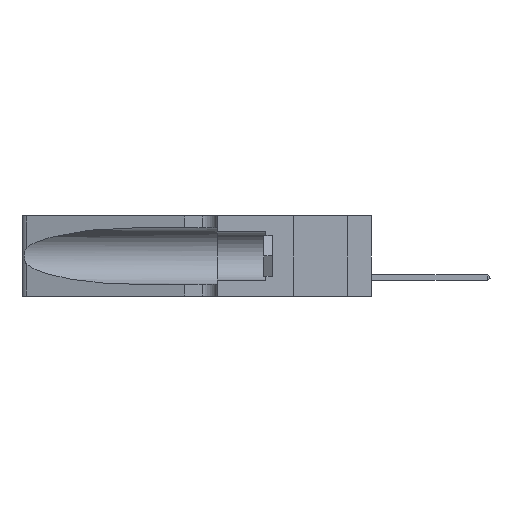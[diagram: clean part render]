
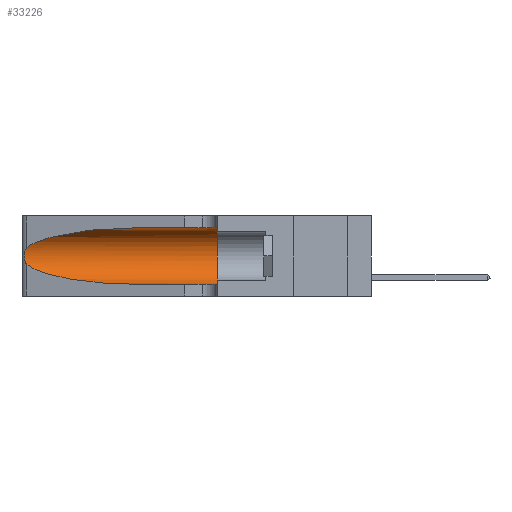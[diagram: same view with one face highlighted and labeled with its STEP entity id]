
A CAD part, left-side view. The second image highlights one B-rep face of the part: STEP entity #33226.
In plain terms, the highlighted cylindrical face has radius 3.308 mm (diameter 6.617 mm), a partial arc.
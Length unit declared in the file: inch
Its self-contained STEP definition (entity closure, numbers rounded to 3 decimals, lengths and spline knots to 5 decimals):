
#1278 = VERTEX_POINT ( 'NONE', #46199 ) ;
#1448 = CARTESIAN_POINT ( 'NONE',  ( 0.25555, 1.22993, 0.14849 ) ) ;
#1820 = CARTESIAN_POINT ( 'NONE',  ( 0.25555, 1.22994, 0.2215 ) ) ;
#1903 = CARTESIAN_POINT ( 'NONE',  ( 0.2373, 1.15595, 0.08982 ) ) ;
#3109 = CARTESIAN_POINT ( 'NONE',  ( 0.25487, 1.22718, 0.14631 ) ) ;
#5463 = CARTESIAN_POINT ( 'NONE',  ( 0.25789, 1.23486, 0.15765 ) ) ;
#5542 = CARTESIAN_POINT ( 'NONE',  ( 0.25487, 1.22718, 0.22369 ) ) ;
#6098 = VERTEX_POINT ( 'NONE', #3109 ) ;
#6198 = CARTESIAN_POINT ( 'NONE',  ( 0.26075, 1.23896, 0.19203 ) ) ;
#7115 = CARTESIAN_POINT ( 'NONE',  ( 0.25487, 1.22718, 0.22369 ) ) ;
#7576 = VERTEX_POINT ( 'NONE', #30046 ) ;
#7947 = CARTESIAN_POINT ( 'NONE',  ( 0.1305, 1.61858, 0.31525 ) ) ;
#8960 = ORIENTED_EDGE ( 'NONE', *, *, #21991, .T. ) ;
#10146 = CARTESIAN_POINT ( 'NONE',  ( 0.26075, 1.23896, 0.178 ) ) ;
#12109 = DIRECTION ( 'NONE',  ( 0., 1., 0. ) ) ;
#12801 = EDGE_CURVE ( 'NONE', #7576, #27896, #23315, .T. ) ;
#13102 = ORIENTED_EDGE ( 'NONE', *, *, #45933, .F. ) ;
#13615 = DIRECTION ( 'NONE',  ( 0., 0., -1. ) ) ;
#14048 = CARTESIAN_POINT ( 'NONE',  ( 0.25487, 1.22718, 0.22369 ) ) ;
#16147 = CARTESIAN_POINT ( 'NONE',  ( 0.1305, 0.72297, 0.31525 ) ) ;
#16413 = EDGE_CURVE ( 'NONE', #36923, #6098, #18307, .T. ) ;
#17496 = LINE ( 'NONE', #32997, #35770 ) ;
#17593 = CARTESIAN_POINT ( 'NONE',  ( 0.25487, 1.22718, 0.14631 ) ) ;
#17693 = CARTESIAN_POINT ( 'NONE',  ( 0.1305, 0.72297, 0.05475 ) ) ;
#17925 = ORIENTED_EDGE ( 'NONE', *, *, #24332, .T. ) ;
#18108 = AXIS2_PLACEMENT_3D ( 'NONE', #21817, #29509, #13615 ) ;
#18307 = B_SPLINE_CURVE_WITH_KNOTS ( 'NONE', 3,
 ( #14048, #1820, #48616, #25441, #40738, #21310, #6198, #10146, #36994, #24883, #5463, #29008, #1448, #17593 ),
 .UNSPECIFIED., .F., .F.,
 ( 4, 2, 2, 2, 2, 2, 4 ),
 ( 0., 0.00027, 0.00053, 0.00107, 0.0016, 0.00187, 0.00214 ),
 .UNSPECIFIED. ) ;
#21310 = CARTESIAN_POINT ( 'NONE',  ( 0.26018, 1.23835, 0.19895 ) ) ;
#21817 = CARTESIAN_POINT ( 'NONE',  ( 0.1305, 1.61858, 0.185 ) ) ;
#21991 = EDGE_CURVE ( 'NONE', #7576, #36923, #24429, .T. ) ;
#23315 = LINE ( 'NONE', #7947, #39701 ) ;
#24133 = DIRECTION ( 'NONE',  ( 0., 0., 1. ) ) ;
#24332 = EDGE_CURVE ( 'NONE', #6098, #1278, #41738, .T. ) ;
#24429 =( BOUNDED_CURVE ( )  B_SPLINE_CURVE ( 3, ( #16147, #43410, #40473, #5542 ),
 .UNSPECIFIED., .F., .F. ) 
 B_SPLINE_CURVE_WITH_KNOTS ( ( 4, 4 ),
 ( 1.5708, 2.84003 ),
 .UNSPECIFIED. ) 
 CURVE ( )  GEOMETRIC_REPRESENTATION_ITEM ( )  RATIONAL_B_SPLINE_CURVE ( ( 1., 0.87, 0.87, 1. ) ) 
 REPRESENTATION_ITEM ( '' )  );
#24883 = CARTESIAN_POINT ( 'NONE',  ( 0.25856, 1.23593, 0.16098 ) ) ;
#25441 = CARTESIAN_POINT ( 'NONE',  ( 0.25787, 1.23484, 0.2124 ) ) ;
#27577 = CARTESIAN_POINT ( 'NONE',  ( 0.1305, 0.35, 0.185 ) ) ;
#27896 = VERTEX_POINT ( 'NONE', #44092 ) ;
#28543 = CARTESIAN_POINT ( 'NONE',  ( 0.18966, 0.96281, 0.05475 ) ) ;
#29008 = CARTESIAN_POINT ( 'NONE',  ( 0.25639, 1.23186, 0.15144 ) ) ;
#29509 = DIRECTION ( 'NONE',  ( 0., -1., 0. ) ) ;
#30046 = CARTESIAN_POINT ( 'NONE',  ( 0.1305, 0.72297, 0.31525 ) ) ;
#30147 = CIRCLE ( 'NONE', #42010, 0.13025 ) ;
#30459 = ORIENTED_EDGE ( 'NONE', *, *, #12801, .F. ) ;
#32315 = DIRECTION ( 'NONE',  ( 0., -1., 0. ) ) ;
#32997 = CARTESIAN_POINT ( 'NONE',  ( 0.1305, 1.61858, 0.05475 ) ) ;
#33226 = ADVANCED_FACE ( 'NONE', ( #49465 ), #34217, .F. ) ;
#34217 = CYLINDRICAL_SURFACE ( 'NONE', #18108, 0.13025 ) ;
#35145 = VERTEX_POINT ( 'NONE', #50354 ) ;
#35770 = VECTOR ( 'NONE', #32315, 39.37008 ) ;
#36923 = VERTEX_POINT ( 'NONE', #7115 ) ;
#36994 = CARTESIAN_POINT ( 'NONE',  ( 0.26017, 1.23833, 0.17102 ) ) ;
#38183 = ORIENTED_EDGE ( 'NONE', *, *, #49529, .T. ) ;
#39701 = VECTOR ( 'NONE', #50303, 39.37008 ) ;
#40473 = CARTESIAN_POINT ( 'NONE',  ( 0.2373, 1.15595, 0.28018 ) ) ;
#40738 = CARTESIAN_POINT ( 'NONE',  ( 0.25854, 1.2359, 0.20912 ) ) ;
#41738 =( BOUNDED_CURVE ( )  B_SPLINE_CURVE ( 3, ( #44984, #1903, #28543, #17693 ),
 .UNSPECIFIED., .F., .T. ) 
 B_SPLINE_CURVE_WITH_KNOTS ( ( 4, 4 ),
 ( 3.44316, 4.71239 ),
 .UNSPECIFIED. ) 
 CURVE ( )  GEOMETRIC_REPRESENTATION_ITEM ( )  RATIONAL_B_SPLINE_CURVE ( ( 1., 0.87, 0.87, 1. ) ) 
 REPRESENTATION_ITEM ( '' )  );
#42010 = AXIS2_PLACEMENT_3D ( 'NONE', #27577, #12109, #24133 ) ;
#43410 = CARTESIAN_POINT ( 'NONE',  ( 0.18966, 0.96281, 0.31525 ) ) ;
#44092 = CARTESIAN_POINT ( 'NONE',  ( 0.1305, 0.35, 0.31525 ) ) ;
#44984 = CARTESIAN_POINT ( 'NONE',  ( 0.25487, 1.22718, 0.14631 ) ) ;
#45933 = EDGE_CURVE ( 'NONE', #27896, #35145, #30147, .T. ) ;
#46199 = CARTESIAN_POINT ( 'NONE',  ( 0.1305, 0.72297, 0.05475 ) ) ;
#48033 = EDGE_LOOP ( 'NONE', ( #8960, #49123, #17925, #38183, #13102, #30459 ) ) ;
#48616 = CARTESIAN_POINT ( 'NONE',  ( 0.25639, 1.23184, 0.21858 ) ) ;
#49123 = ORIENTED_EDGE ( 'NONE', *, *, #16413, .T. ) ;
#49465 = FACE_OUTER_BOUND ( 'NONE', #48033, .T. ) ;
#49529 = EDGE_CURVE ( 'NONE', #1278, #35145, #17496, .T. ) ;
#50303 = DIRECTION ( 'NONE',  ( 0., -1., 0. ) ) ;
#50354 = CARTESIAN_POINT ( 'NONE',  ( 0.1305, 0.35, 0.05475 ) ) ;
